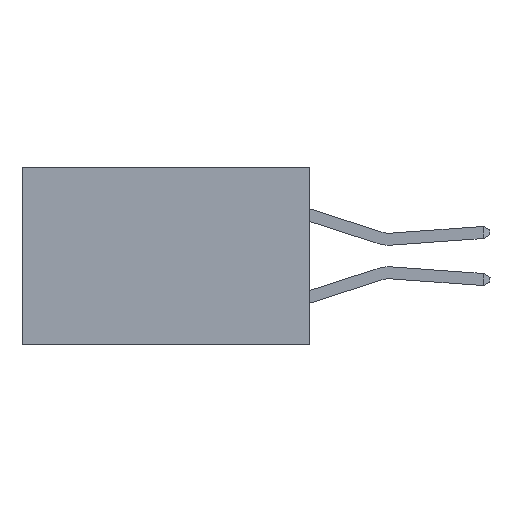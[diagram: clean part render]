
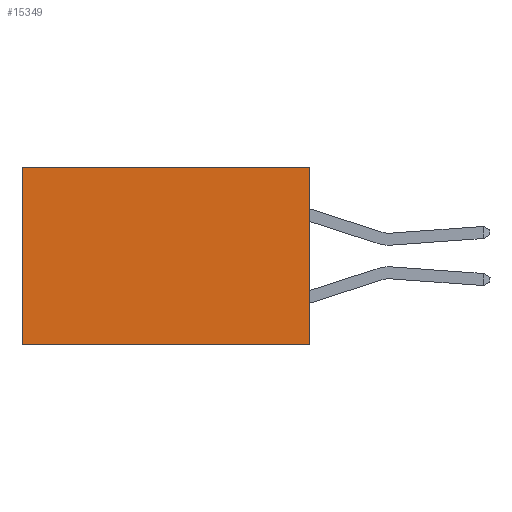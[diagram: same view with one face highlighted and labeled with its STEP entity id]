
A CAD part, left-side view. The second image highlights one B-rep face of the part: STEP entity #15349.
In plain terms, the highlighted planar face has unit normal (-1, 0, 0).
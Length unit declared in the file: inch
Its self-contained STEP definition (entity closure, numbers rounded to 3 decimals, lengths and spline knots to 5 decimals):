
#81 = CARTESIAN_POINT ( 'NONE',  ( 0.298, 0., 0. ) ) ;
#887 = CARTESIAN_POINT ( 'NONE',  ( 0.298, 0.6, 0. ) ) ;
#1045 = VECTOR ( 'NONE', #15697, 39.37008 ) ;
#1533 = DIRECTION ( 'NONE',  ( 0., 0., -1. ) ) ;
#2331 = CARTESIAN_POINT ( 'NONE',  ( 0.298, 0., 0. ) ) ;
#4135 = EDGE_CURVE ( 'NONE', #6655, #14484, #18068, .T. ) ;
#4595 = EDGE_CURVE ( 'NONE', #6655, #13957, #15687, .T. ) ;
#5240 = CARTESIAN_POINT ( 'NONE',  ( 0.298, 0., -0.37 ) ) ;
#5618 = DIRECTION ( 'NONE',  ( 0., 1., 0. ) ) ;
#6493 = VECTOR ( 'NONE', #1533, 39.37008 ) ;
#6655 = VERTEX_POINT ( 'NONE', #81 ) ;
#6707 = EDGE_LOOP ( 'NONE', ( #11891, #13035, #12258, #9759 ) ) ;
#7200 = DIRECTION ( 'NONE',  ( 1., 0., 0. ) ) ;
#7365 = VERTEX_POINT ( 'NONE', #18615 ) ;
#8786 = LINE ( 'NONE', #18658, #1045 ) ;
#8843 = DIRECTION ( 'NONE',  ( 0., 0., -1. ) ) ;
#9559 = LINE ( 'NONE', #15105, #6493 ) ;
#9759 = ORIENTED_EDGE ( 'NONE', *, *, #4135, .T. ) ;
#10357 = VECTOR ( 'NONE', #5618, 39.37008 ) ;
#10362 = PLANE ( 'NONE',  #13188 ) ;
#11891 = ORIENTED_EDGE ( 'NONE', *, *, #17564, .T. ) ;
#12258 = ORIENTED_EDGE ( 'NONE', *, *, #4595, .F. ) ;
#13035 = ORIENTED_EDGE ( 'NONE', *, *, #18856, .F. ) ;
#13188 = AXIS2_PLACEMENT_3D ( 'NONE', #16172, #7200, #13337 ) ;
#13337 = DIRECTION ( 'NONE',  ( 0., 0., -1. ) ) ;
#13957 = VERTEX_POINT ( 'NONE', #5240 ) ;
#14073 = FACE_OUTER_BOUND ( 'NONE', #6707, .T. ) ;
#14484 = VERTEX_POINT ( 'NONE', #887 ) ;
#15105 = CARTESIAN_POINT ( 'NONE',  ( 0.298, 0.6, 0. ) ) ;
#15349 = ADVANCED_FACE ( 'NONE', ( #14073 ), #10362, .F. ) ;
#15687 = LINE ( 'NONE', #17628, #15930 ) ;
#15697 = DIRECTION ( 'NONE',  ( 0., 1., 0. ) ) ;
#15930 = VECTOR ( 'NONE', #8843, 39.37008 ) ;
#16172 = CARTESIAN_POINT ( 'NONE',  ( 0.298, 0., 0. ) ) ;
#17564 = EDGE_CURVE ( 'NONE', #14484, #7365, #9559, .T. ) ;
#17628 = CARTESIAN_POINT ( 'NONE',  ( 0.298, 0., 0. ) ) ;
#18068 = LINE ( 'NONE', #2331, #10357 ) ;
#18615 = CARTESIAN_POINT ( 'NONE',  ( 0.298, 0.6, -0.37 ) ) ;
#18658 = CARTESIAN_POINT ( 'NONE',  ( 0.298, 0., -0.37 ) ) ;
#18856 = EDGE_CURVE ( 'NONE', #13957, #7365, #8786, .T. ) ;
